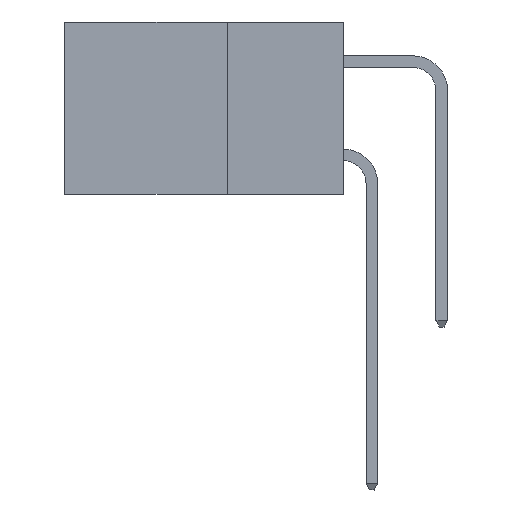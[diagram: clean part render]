
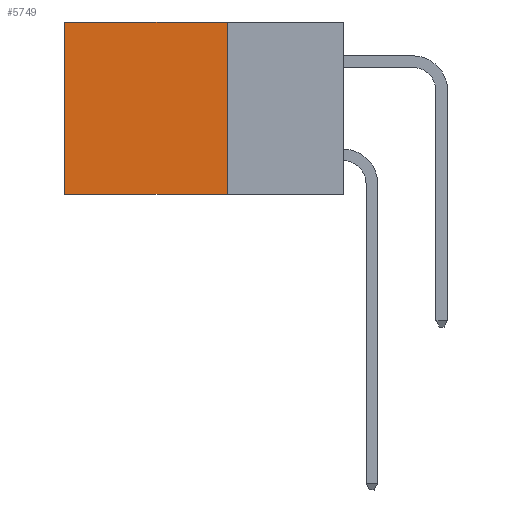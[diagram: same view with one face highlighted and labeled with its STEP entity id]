
A CAD part, left-side view. The second image highlights one B-rep face of the part: STEP entity #5749.
In plain terms, the highlighted planar face has unit normal (-1, 0, 0).
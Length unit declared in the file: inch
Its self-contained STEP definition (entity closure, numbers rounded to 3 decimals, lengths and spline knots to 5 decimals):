
#854 = CARTESIAN_POINT ( 'NONE',  ( 0.298, 0.25, 0. ) ) ;
#2625 = EDGE_CURVE ( 'NONE', #27706, #9008, #27918, .T. ) ;
#3557 = VERTEX_POINT ( 'NONE', #19885 ) ;
#5749 = ADVANCED_FACE ( 'NONE', ( #9793 ), #23055, .F. ) ;
#6280 = CARTESIAN_POINT ( 'NONE',  ( 0.298, 0.25, 0. ) ) ;
#6791 = DIRECTION ( 'NONE',  ( 0., 1., 0. ) ) ;
#8285 = ORIENTED_EDGE ( 'NONE', *, *, #29361, .T. ) ;
#8381 = DIRECTION ( 'NONE',  ( 1., 0., 0. ) ) ;
#8658 = EDGE_CURVE ( 'NONE', #3557, #12060, #24395, .T. ) ;
#9008 = VERTEX_POINT ( 'NONE', #17375 ) ;
#9793 = FACE_OUTER_BOUND ( 'NONE', #21964, .T. ) ;
#10009 = VECTOR ( 'NONE', #16582, 39.37008 ) ;
#10164 = ORIENTED_EDGE ( 'NONE', *, *, #14039, .F. ) ;
#11414 = VECTOR ( 'NONE', #13757, 39.37008 ) ;
#12060 = VERTEX_POINT ( 'NONE', #14082 ) ;
#12137 = AXIS2_PLACEMENT_3D ( 'NONE', #854, #8381, #25461 ) ;
#13450 = VECTOR ( 'NONE', #6791, 39.37008 ) ;
#13732 = ORIENTED_EDGE ( 'NONE', *, *, #2625, .T. ) ;
#13757 = DIRECTION ( 'NONE',  ( 0., 0., -1. ) ) ;
#14039 = EDGE_CURVE ( 'NONE', #12060, #9008, #27140, .T. ) ;
#14082 = CARTESIAN_POINT ( 'NONE',  ( 0.298, 0.25, -0.37 ) ) ;
#16582 = DIRECTION ( 'NONE',  ( 0., 0., -1. ) ) ;
#17375 = CARTESIAN_POINT ( 'NONE',  ( 0.298, 0.6, -0.37 ) ) ;
#17438 = VECTOR ( 'NONE', #25783, 39.37008 ) ;
#17749 = CARTESIAN_POINT ( 'NONE',  ( 0.298, 0.6, 0. ) ) ;
#18185 = LINE ( 'NONE', #30629, #17438 ) ;
#19885 = CARTESIAN_POINT ( 'NONE',  ( 0.298, 0.25, 0. ) ) ;
#21964 = EDGE_LOOP ( 'NONE', ( #13732, #10164, #29360, #8285 ) ) ;
#23055 = PLANE ( 'NONE',  #12137 ) ;
#23946 = CARTESIAN_POINT ( 'NONE',  ( 0.298, 0.25, -0.37 ) ) ;
#24395 = LINE ( 'NONE', #6280, #11414 ) ;
#25461 = DIRECTION ( 'NONE',  ( 0., 0., -1. ) ) ;
#25783 = DIRECTION ( 'NONE',  ( 0., 1., 0. ) ) ;
#26203 = CARTESIAN_POINT ( 'NONE',  ( 0.298, 0.6, 0. ) ) ;
#27140 = LINE ( 'NONE', #23946, #13450 ) ;
#27706 = VERTEX_POINT ( 'NONE', #17749 ) ;
#27918 = LINE ( 'NONE', #26203, #10009 ) ;
#29360 = ORIENTED_EDGE ( 'NONE', *, *, #8658, .F. ) ;
#29361 = EDGE_CURVE ( 'NONE', #3557, #27706, #18185, .T. ) ;
#30629 = CARTESIAN_POINT ( 'NONE',  ( 0.298, 0.25, 0. ) ) ;
